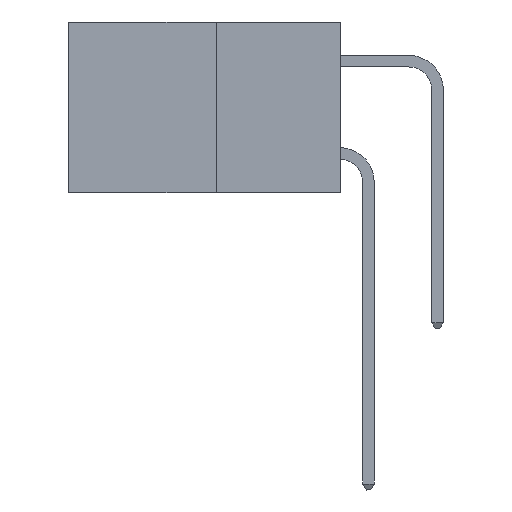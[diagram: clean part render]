
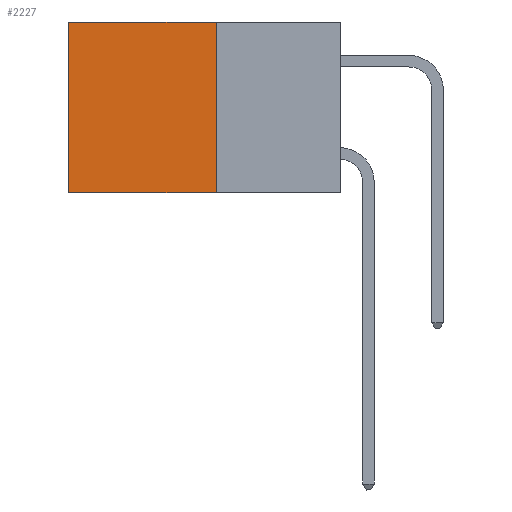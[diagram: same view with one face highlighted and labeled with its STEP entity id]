
A CAD part, left-side view. The second image highlights one B-rep face of the part: STEP entity #2227.
In plain terms, the highlighted planar face has unit normal (-1, 0, 0).
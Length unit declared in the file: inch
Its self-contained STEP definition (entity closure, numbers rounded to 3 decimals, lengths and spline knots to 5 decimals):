
#403 = DIRECTION ( 'NONE',  ( 0., 1., 0. ) ) ;
#1272 = EDGE_CURVE ( 'NONE', #8377, #4047, #6666, .T. ) ;
#2227 = ADVANCED_FACE ( 'NONE', ( #13439 ), #7907, .F. ) ;
#2269 = VECTOR ( 'NONE', #13217, 39.37008 ) ;
#2364 = ORIENTED_EDGE ( 'NONE', *, *, #14593, .T. ) ;
#2395 = CARTESIAN_POINT ( 'NONE',  ( 0.277, 0.27, -0.37 ) ) ;
#3128 = EDGE_LOOP ( 'NONE', ( #4094, #13562, #8971, #2364 ) ) ;
#3157 = CARTESIAN_POINT ( 'NONE',  ( 0.277, 0.27, -0.37 ) ) ;
#3471 = VECTOR ( 'NONE', #8052, 39.37008 ) ;
#3478 = VECTOR ( 'NONE', #8844, 39.37008 ) ;
#4047 = VERTEX_POINT ( 'NONE', #13920 ) ;
#4094 = ORIENTED_EDGE ( 'NONE', *, *, #1272, .T. ) ;
#6666 = LINE ( 'NONE', #14327, #3478 ) ;
#6813 = CARTESIAN_POINT ( 'NONE',  ( 0.277, 0.27, -0.37 ) ) ;
#7358 = EDGE_CURVE ( 'NONE', #14212, #4047, #12330, .T. ) ;
#7907 = PLANE ( 'NONE',  #13858 ) ;
#8052 = DIRECTION ( 'NONE',  ( 0., 0., -1. ) ) ;
#8377 = VERTEX_POINT ( 'NONE', #15244 ) ;
#8844 = DIRECTION ( 'NONE',  ( 0., 0., -1. ) ) ;
#8892 = CARTESIAN_POINT ( 'NONE',  ( 0.277, 0.27, 0. ) ) ;
#8971 = ORIENTED_EDGE ( 'NONE', *, *, #12095, .F. ) ;
#9430 = CARTESIAN_POINT ( 'NONE',  ( 0.277, 0.27, 0. ) ) ;
#9535 = DIRECTION ( 'NONE',  ( 0., 0., -1. ) ) ;
#9537 = DIRECTION ( 'NONE',  ( 1., 0., 0. ) ) ;
#10994 = VERTEX_POINT ( 'NONE', #9430 ) ;
#12095 = EDGE_CURVE ( 'NONE', #10994, #14212, #13110, .T. ) ;
#12330 = LINE ( 'NONE', #2395, #2269 ) ;
#12490 = LINE ( 'NONE', #8892, #12857 ) ;
#12610 = CARTESIAN_POINT ( 'NONE',  ( 0.277, 0.27, -0.37 ) ) ;
#12857 = VECTOR ( 'NONE', #403, 39.37008 ) ;
#13110 = LINE ( 'NONE', #6813, #3471 ) ;
#13217 = DIRECTION ( 'NONE',  ( 0., 1., 0. ) ) ;
#13439 = FACE_OUTER_BOUND ( 'NONE', #3128, .T. ) ;
#13562 = ORIENTED_EDGE ( 'NONE', *, *, #7358, .F. ) ;
#13858 = AXIS2_PLACEMENT_3D ( 'NONE', #12610, #9537, #9535 ) ;
#13920 = CARTESIAN_POINT ( 'NONE',  ( 0.277, 0.59, -0.37 ) ) ;
#14212 = VERTEX_POINT ( 'NONE', #3157 ) ;
#14327 = CARTESIAN_POINT ( 'NONE',  ( 0.277, 0.59, -0.37 ) ) ;
#14593 = EDGE_CURVE ( 'NONE', #10994, #8377, #12490, .T. ) ;
#15244 = CARTESIAN_POINT ( 'NONE',  ( 0.277, 0.59, 0. ) ) ;
